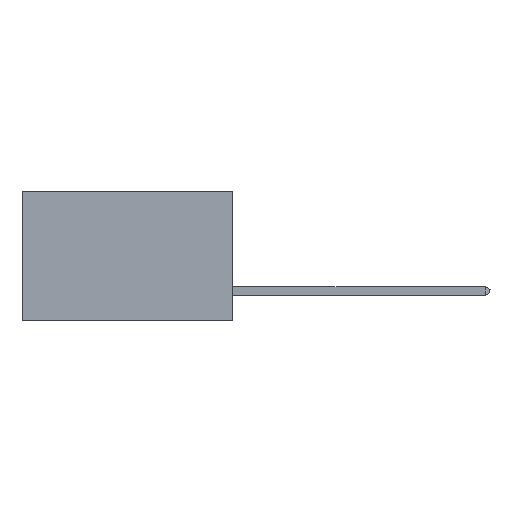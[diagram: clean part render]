
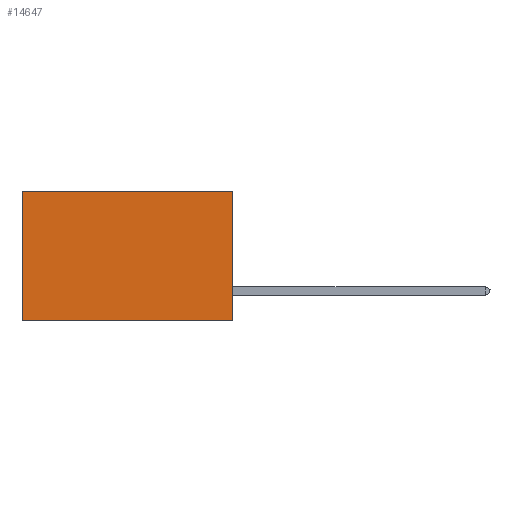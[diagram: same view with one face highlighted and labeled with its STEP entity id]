
A CAD part, left-side view. The second image highlights one B-rep face of the part: STEP entity #14647.
In plain terms, the highlighted planar face has unit normal (-1, 0, 0).
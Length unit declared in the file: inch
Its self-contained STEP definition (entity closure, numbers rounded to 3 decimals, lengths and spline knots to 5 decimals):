
#215 = VERTEX_POINT ( 'NONE', #37881 ) ;
#453 = ORIENTED_EDGE ( 'NONE', *, *, #46190, .T. ) ;
#2009 = CARTESIAN_POINT ( 'NONE',  ( 0.2875, 0., 0. ) ) ;
#5719 = DIRECTION ( 'NONE',  ( 0., 0., -1. ) ) ;
#6361 = EDGE_LOOP ( 'NONE', ( #34314, #24584, #47141, #453 ) ) ;
#11357 = DIRECTION ( 'NONE',  ( 0., 0., -1. ) ) ;
#11726 = AXIS2_PLACEMENT_3D ( 'NONE', #2009, #27837, #5719 ) ;
#11954 = DIRECTION ( 'NONE',  ( 0., 1., 0. ) ) ;
#12542 = LINE ( 'NONE', #44123, #40916 ) ;
#12837 = LINE ( 'NONE', #33500, #20348 ) ;
#13794 = FACE_OUTER_BOUND ( 'NONE', #6361, .T. ) ;
#14647 = ADVANCED_FACE ( 'NONE', ( #13794 ), #42614, .F. ) ;
#19010 = VERTEX_POINT ( 'NONE', #47598 ) ;
#20329 = DIRECTION ( 'NONE',  ( 0., 0., -1. ) ) ;
#20348 = VECTOR ( 'NONE', #11357, 39.37008 ) ;
#20562 = LINE ( 'NONE', #42532, #31562 ) ;
#21637 = LINE ( 'NONE', #44944, #46562 ) ;
#22882 = CARTESIAN_POINT ( 'NONE',  ( 0.2875, 0.6, 0. ) ) ;
#24402 = CARTESIAN_POINT ( 'NONE',  ( 0.2875, 0.6, -0.37 ) ) ;
#24584 = ORIENTED_EDGE ( 'NONE', *, *, #29637, .F. ) ;
#27837 = DIRECTION ( 'NONE',  ( 1., 0., 0. ) ) ;
#29637 = EDGE_CURVE ( 'NONE', #19010, #41720, #21637, .T. ) ;
#31353 = EDGE_CURVE ( 'NONE', #215, #19010, #20562, .T. ) ;
#31562 = VECTOR ( 'NONE', #20329, 39.37008 ) ;
#33317 = EDGE_CURVE ( 'NONE', #36054, #41720, #12837, .T. ) ;
#33500 = CARTESIAN_POINT ( 'NONE',  ( 0.2875, 0.6, 0. ) ) ;
#34314 = ORIENTED_EDGE ( 'NONE', *, *, #33317, .T. ) ;
#36054 = VERTEX_POINT ( 'NONE', #22882 ) ;
#36679 = DIRECTION ( 'NONE',  ( 0., 1., 0. ) ) ;
#37881 = CARTESIAN_POINT ( 'NONE',  ( 0.2875, 0., 0. ) ) ;
#40916 = VECTOR ( 'NONE', #36679, 39.37008 ) ;
#41720 = VERTEX_POINT ( 'NONE', #24402 ) ;
#42532 = CARTESIAN_POINT ( 'NONE',  ( 0.2875, 0., 0. ) ) ;
#42614 = PLANE ( 'NONE',  #11726 ) ;
#44123 = CARTESIAN_POINT ( 'NONE',  ( 0.2875, 0., 0. ) ) ;
#44944 = CARTESIAN_POINT ( 'NONE',  ( 0.2875, 0., -0.37 ) ) ;
#46190 = EDGE_CURVE ( 'NONE', #215, #36054, #12542, .T. ) ;
#46562 = VECTOR ( 'NONE', #11954, 39.37008 ) ;
#47141 = ORIENTED_EDGE ( 'NONE', *, *, #31353, .F. ) ;
#47598 = CARTESIAN_POINT ( 'NONE',  ( 0.2875, 0., -0.37 ) ) ;
